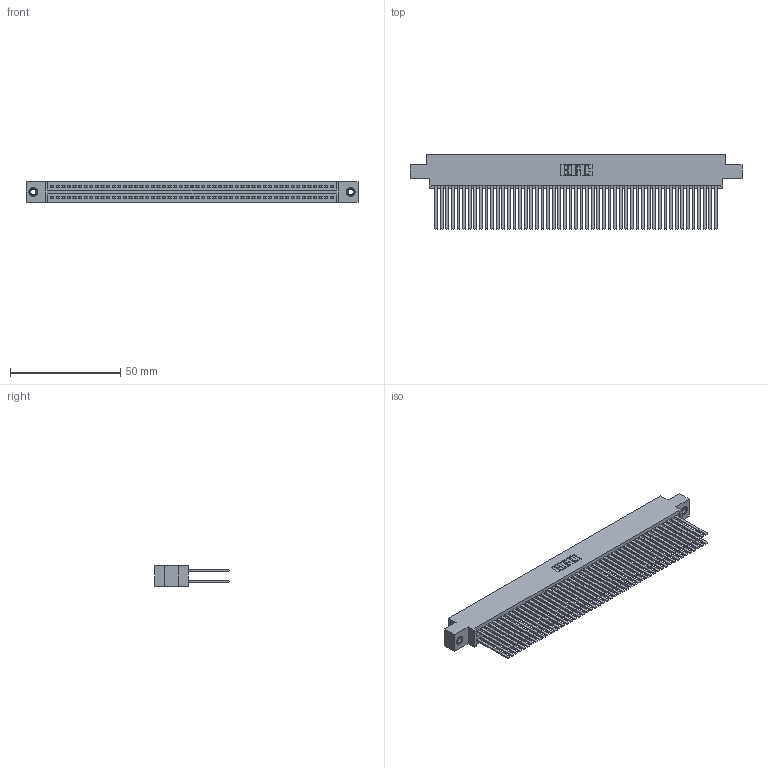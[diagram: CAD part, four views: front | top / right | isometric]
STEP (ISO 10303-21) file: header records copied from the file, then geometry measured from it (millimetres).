
FILE_DESCRIPTION (( 'STEP AP203' ), '1' );
FILE_NAME ('345-102-544-807.STEP', '2019-11-03T08:36:56', ( '' ), ( '' ), 'SwSTEP 2.0', 'SolidWorks 2016', '' );
FILE_SCHEMA (( 'CONFIG_CONTROL_DESIGN' ));
Length unit declared in the file: inch
Products named in the file (4): 345-250-001_345-250-005-103; 345-102-544-807; 345 Part_0.170 Offset - 0.156 Dia-TI; 345-292-001_345-293-144
Assembly tree (105 placements, depth 2):
  345-102-544-807
    345 Part_0.170 Offset - 0.156 Dia-TI
    345-292-001_345-293-144  x102
    345-250-001_345-250-005-103  x2
Bounding box: 150.75 x 33.96 x 9.4 mm (x, y, z)
Volume: 16030.4 mm3; surface area: 28232.1 mm2
Topology: 105 solids, 105 shells, 4678 faces, 13851 edges, 9090 vertices
Faces by surface type: plane 3074, cylinder 1588, cone 12, torus 4
Entity records: 39938 total; most frequent: CARTESIAN_POINT 6667, ORIENTED_EDGE 6594, DIRECTION 5891, EDGE_CURVE 3297, VECTOR 2945, LINE 2945, VERTEX_POINT 2192, AXIS2_PLACEMENT_3D 1473
